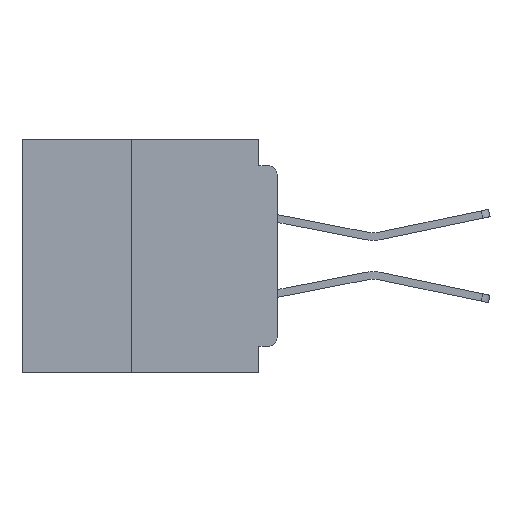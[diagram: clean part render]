
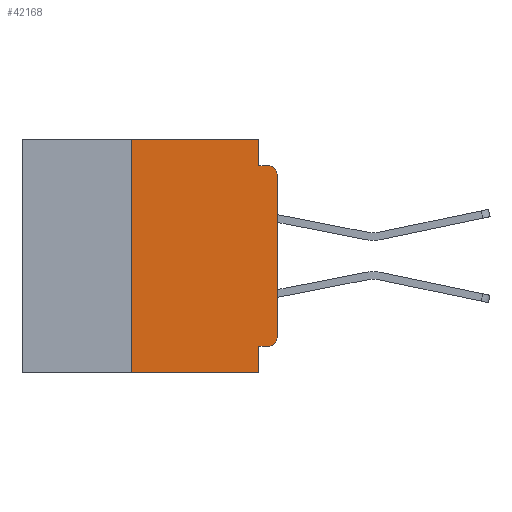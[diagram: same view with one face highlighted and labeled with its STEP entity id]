
A CAD part, left-side view. The second image highlights one B-rep face of the part: STEP entity #42168.
In plain terms, the highlighted planar face has unit normal (-1, 0, 0).
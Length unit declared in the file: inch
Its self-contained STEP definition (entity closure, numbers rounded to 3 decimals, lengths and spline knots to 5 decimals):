
#693 = EDGE_LOOP ( 'NONE', ( #8340, #19718, #33305, #31797, #45840, #21205, #39975, #19118, #21366, #6611 ) ) ;
#890 = EDGE_CURVE ( 'NONE', #12796, #40134, #19474, .T. ) ;
#1226 = CARTESIAN_POINT ( 'NONE',  ( 0., 0.031, -0.4 ) ) ;
#1856 = AXIS2_PLACEMENT_3D ( 'NONE', #20008, #36533, #11867 ) ;
#1878 = CARTESIAN_POINT ( 'NONE',  ( 0., 0.031, -0.355 ) ) ;
#1920 = VECTOR ( 'NONE', #34808, 39.37008 ) ;
#2492 = DIRECTION ( 'NONE',  ( -1., 0., 0. ) ) ;
#3634 = DIRECTION ( 'NONE',  ( 0., 0., -1. ) ) ;
#3872 = DIRECTION ( 'NONE',  ( 0., -1., 0. ) ) ;
#4865 = CARTESIAN_POINT ( 'NONE',  ( 0., 0.015, -0.045 ) ) ;
#5453 = DIRECTION ( 'NONE',  ( 0., 0., -1. ) ) ;
#6611 = ORIENTED_EDGE ( 'NONE', *, *, #30039, .T. ) ;
#6751 = EDGE_CURVE ( 'NONE', #40134, #15796, #13050, .T. ) ;
#6993 = FACE_OUTER_BOUND ( 'NONE', #693, .T. ) ;
#7551 = EDGE_CURVE ( 'NONE', #43984, #23394, #37433, .T. ) ;
#8340 = ORIENTED_EDGE ( 'NONE', *, *, #46093, .T. ) ;
#8439 = CIRCLE ( 'NONE', #33251, 0.015 ) ;
#10985 = LINE ( 'NONE', #21319, #42432 ) ;
#11867 = DIRECTION ( 'NONE',  ( 0., 0., -1. ) ) ;
#12593 = CARTESIAN_POINT ( 'NONE',  ( 0., 0., -0.355 ) ) ;
#12796 = VERTEX_POINT ( 'NONE', #42588 ) ;
#13050 = LINE ( 'NONE', #18430, #1920 ) ;
#13188 = DIRECTION ( 'NONE',  ( 0., 0., 1. ) ) ;
#13573 = VECTOR ( 'NONE', #49126, 39.37008 ) ;
#14907 = LINE ( 'NONE', #49146, #47533 ) ;
#14958 = CARTESIAN_POINT ( 'NONE',  ( 0., 0., 0. ) ) ;
#15552 = VECTOR ( 'NONE', #5453, 39.37008 ) ;
#15796 = VERTEX_POINT ( 'NONE', #26160 ) ;
#17699 = CIRCLE ( 'NONE', #45822, 0.015 ) ;
#18178 = VECTOR ( 'NONE', #46985, 39.37008 ) ;
#18430 = CARTESIAN_POINT ( 'NONE',  ( 0., 0.031, 0. ) ) ;
#19118 = ORIENTED_EDGE ( 'NONE', *, *, #7551, .F. ) ;
#19474 = LINE ( 'NONE', #43251, #18178 ) ;
#19638 = VECTOR ( 'NONE', #29165, 39.37008 ) ;
#19718 = ORIENTED_EDGE ( 'NONE', *, *, #29483, .T. ) ;
#20008 = CARTESIAN_POINT ( 'NONE',  ( 0., 0.437, 0. ) ) ;
#21146 = EDGE_CURVE ( 'NONE', #37302, #43984, #30593, .T. ) ;
#21205 = ORIENTED_EDGE ( 'NONE', *, *, #41669, .F. ) ;
#21319 = CARTESIAN_POINT ( 'NONE',  ( 0., 0.25, -0.4 ) ) ;
#21366 = ORIENTED_EDGE ( 'NONE', *, *, #21146, .F. ) ;
#23252 = EDGE_CURVE ( 'NONE', #44728, #23394, #46243, .T. ) ;
#23394 = VERTEX_POINT ( 'NONE', #25427 ) ;
#23597 = CARTESIAN_POINT ( 'NONE',  ( 0., 0.25, -0.4 ) ) ;
#25427 = CARTESIAN_POINT ( 'NONE',  ( 0., 0.031, -0.4 ) ) ;
#26160 = CARTESIAN_POINT ( 'NONE',  ( 0., 0.031, -0.045 ) ) ;
#27329 = CARTESIAN_POINT ( 'NONE',  ( 0., 0.015, -0.34 ) ) ;
#28195 = VERTEX_POINT ( 'NONE', #47965 ) ;
#28450 = DIRECTION ( 'NONE',  ( -1., 0., 0. ) ) ;
#29165 = DIRECTION ( 'NONE',  ( 0., 1., 0. ) ) ;
#29483 = EDGE_CURVE ( 'NONE', #35807, #33710, #8439, .T. ) ;
#30039 = EDGE_CURVE ( 'NONE', #37302, #28195, #17699, .T. ) ;
#30593 = LINE ( 'NONE', #12593, #19638 ) ;
#31491 = DIRECTION ( 'NONE',  ( 0., 0., -1. ) ) ;
#31530 = DIRECTION ( 'NONE',  ( 0., 0., 1. ) ) ;
#31797 = ORIENTED_EDGE ( 'NONE', *, *, #6751, .F. ) ;
#32078 = CARTESIAN_POINT ( 'NONE',  ( 0., 0.031, 0. ) ) ;
#32426 = PLANE ( 'NONE',  #1856 ) ;
#33251 = AXIS2_PLACEMENT_3D ( 'NONE', #52781, #28450, #3634 ) ;
#33305 = ORIENTED_EDGE ( 'NONE', *, *, #49218, .F. ) ;
#33440 = CARTESIAN_POINT ( 'NONE',  ( 0., 0.015, -0.355 ) ) ;
#33710 = VERTEX_POINT ( 'NONE', #4865 ) ;
#34808 = DIRECTION ( 'NONE',  ( 0., 0., -1. ) ) ;
#35807 = VERTEX_POINT ( 'NONE', #44030 ) ;
#36533 = DIRECTION ( 'NONE',  ( 1., 0., 0. ) ) ;
#37302 = VERTEX_POINT ( 'NONE', #33440 ) ;
#37433 = LINE ( 'NONE', #1226, #15552 ) ;
#39975 = ORIENTED_EDGE ( 'NONE', *, *, #23252, .T. ) ;
#40134 = VERTEX_POINT ( 'NONE', #32078 ) ;
#40831 = CARTESIAN_POINT ( 'NONE',  ( 0., 0.437, -0.4 ) ) ;
#41669 = EDGE_CURVE ( 'NONE', #44728, #12796, #10985, .T. ) ;
#42168 = ADVANCED_FACE ( 'NONE', ( #6993 ), #32426, .F. ) ;
#42432 = VECTOR ( 'NONE', #13188, 39.37008 ) ;
#42588 = CARTESIAN_POINT ( 'NONE',  ( 0., 0.25, 0. ) ) ;
#43251 = CARTESIAN_POINT ( 'NONE',  ( 0., 0.437, 0. ) ) ;
#43984 = VERTEX_POINT ( 'NONE', #1878 ) ;
#44030 = CARTESIAN_POINT ( 'NONE',  ( 0., 0., -0.06 ) ) ;
#44728 = VERTEX_POINT ( 'NONE', #23597 ) ;
#45822 = AXIS2_PLACEMENT_3D ( 'NONE', #27329, #2492, #31491 ) ;
#45840 = ORIENTED_EDGE ( 'NONE', *, *, #890, .F. ) ;
#46093 = EDGE_CURVE ( 'NONE', #28195, #35807, #50166, .T. ) ;
#46243 = LINE ( 'NONE', #40831, #13573 ) ;
#46985 = DIRECTION ( 'NONE',  ( 0., -1., 0. ) ) ;
#47533 = VECTOR ( 'NONE', #3872, 39.37008 ) ;
#47965 = CARTESIAN_POINT ( 'NONE',  ( 0., 0., -0.34 ) ) ;
#48899 = VECTOR ( 'NONE', #31530, 39.37008 ) ;
#49126 = DIRECTION ( 'NONE',  ( 0., -1., 0. ) ) ;
#49146 = CARTESIAN_POINT ( 'NONE',  ( 0., 0., -0.045 ) ) ;
#49218 = EDGE_CURVE ( 'NONE', #15796, #33710, #14907, .T. ) ;
#50166 = LINE ( 'NONE', #14958, #48899 ) ;
#52781 = CARTESIAN_POINT ( 'NONE',  ( 0., 0.015, -0.06 ) ) ;
